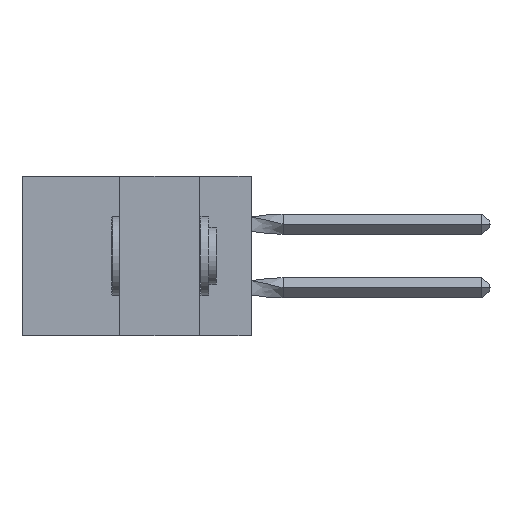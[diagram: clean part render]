
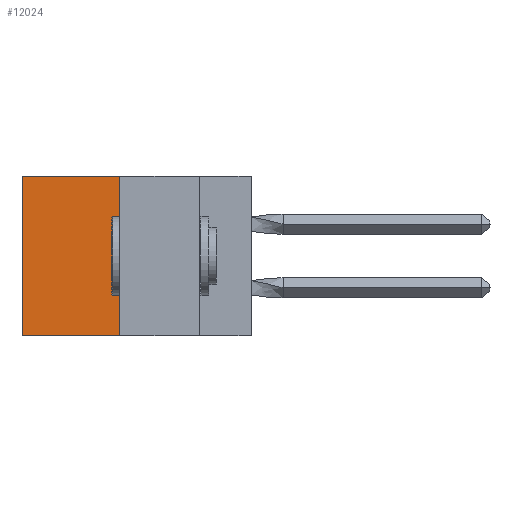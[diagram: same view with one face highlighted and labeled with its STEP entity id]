
A CAD part, left-side view. The second image highlights one B-rep face of the part: STEP entity #12024.
In plain terms, the highlighted planar face has unit normal (-1, 0, 0).
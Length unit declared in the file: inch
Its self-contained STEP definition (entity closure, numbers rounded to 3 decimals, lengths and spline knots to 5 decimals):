
#2748 = EDGE_CURVE ( 'NONE', #23520, #35709, #13824, .T. ) ;
#2933 = LINE ( 'NONE', #29428, #33081 ) ;
#4271 = DIRECTION ( 'NONE',  ( 0., 1., 0. ) ) ;
#4465 = DIRECTION ( 'NONE',  ( 0., 1., 0. ) ) ;
#4646 = CARTESIAN_POINT ( 'NONE',  ( 0.305, 0.413, -0.5 ) ) ;
#4838 = CARTESIAN_POINT ( 'NONE',  ( 0.305, 0.413, -0.5 ) ) ;
#7389 = VECTOR ( 'NONE', #25152, 39.37008 ) ;
#9862 = CARTESIAN_POINT ( 'NONE',  ( 0.305, 0.413, -0.5 ) ) ;
#11492 = ORIENTED_EDGE ( 'NONE', *, *, #29730, .T. ) ;
#12024 = ADVANCED_FACE ( 'NONE', ( #29905 ), #33964, .F. ) ;
#12042 = CARTESIAN_POINT ( 'NONE',  ( 0.305, 0.413, 0. ) ) ;
#13824 = LINE ( 'NONE', #18852, #32569 ) ;
#15438 = ORIENTED_EDGE ( 'NONE', *, *, #36669, .F. ) ;
#15888 = ORIENTED_EDGE ( 'NONE', *, *, #2748, .T. ) ;
#17299 = AXIS2_PLACEMENT_3D ( 'NONE', #4838, #25251, #31110 ) ;
#17882 = ORIENTED_EDGE ( 'NONE', *, *, #36658, .F. ) ;
#18852 = CARTESIAN_POINT ( 'NONE',  ( 0.305, 0.413, 0. ) ) ;
#19036 = CARTESIAN_POINT ( 'NONE',  ( 0.305, 0.413, -0.5 ) ) ;
#23520 = VERTEX_POINT ( 'NONE', #12042 ) ;
#24563 = EDGE_LOOP ( 'NONE', ( #11492, #15438, #17882, #15888 ) ) ;
#25152 = DIRECTION ( 'NONE',  ( 0., 0., -1. ) ) ;
#25251 = DIRECTION ( 'NONE',  ( 1., 0., 0. ) ) ;
#25382 = DIRECTION ( 'NONE',  ( 0., 0., -1. ) ) ;
#26607 = CARTESIAN_POINT ( 'NONE',  ( 0.305, 0.72, -0.5 ) ) ;
#27915 = VERTEX_POINT ( 'NONE', #26607 ) ;
#28034 = CARTESIAN_POINT ( 'NONE',  ( 0.305, 0.72, 0. ) ) ;
#28809 = VECTOR ( 'NONE', #4465, 39.37008 ) ;
#29428 = CARTESIAN_POINT ( 'NONE',  ( 0.305, 0.72, -0.5 ) ) ;
#29730 = EDGE_CURVE ( 'NONE', #35709, #27915, #2933, .T. ) ;
#29905 = FACE_OUTER_BOUND ( 'NONE', #24563, .T. ) ;
#31110 = DIRECTION ( 'NONE',  ( 0., 0., -1. ) ) ;
#31112 = LINE ( 'NONE', #9862, #7389 ) ;
#32569 = VECTOR ( 'NONE', #4271, 39.37008 ) ;
#33081 = VECTOR ( 'NONE', #25382, 39.37008 ) ;
#33236 = VERTEX_POINT ( 'NONE', #4646 ) ;
#33964 = PLANE ( 'NONE',  #17299 ) ;
#35709 = VERTEX_POINT ( 'NONE', #28034 ) ;
#36658 = EDGE_CURVE ( 'NONE', #23520, #33236, #31112, .T. ) ;
#36669 = EDGE_CURVE ( 'NONE', #33236, #27915, #36673, .T. ) ;
#36673 = LINE ( 'NONE', #19036, #28809 ) ;
